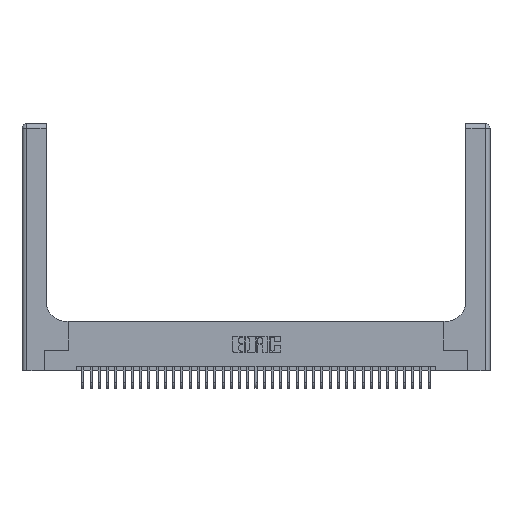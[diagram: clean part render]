
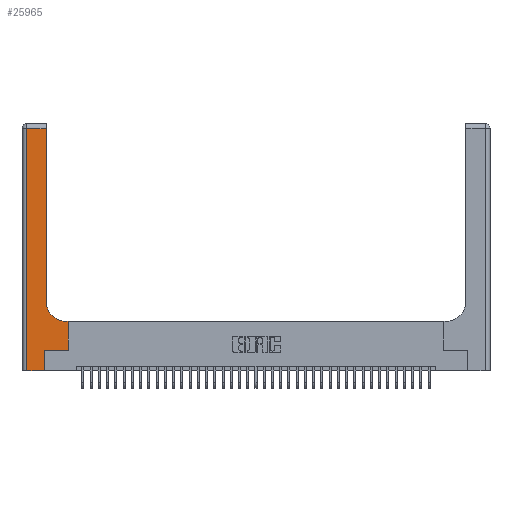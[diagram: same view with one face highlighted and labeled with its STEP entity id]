
A CAD part, top view. The second image highlights one B-rep face of the part: STEP entity #25965.
In plain terms, the highlighted planar face has unit normal (0, 0, 1).
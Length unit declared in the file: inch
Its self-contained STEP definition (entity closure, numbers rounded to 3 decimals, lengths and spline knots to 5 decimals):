
#508 = EDGE_CURVE ( 'NONE', #5268, #9219, #32286, .T. ) ;
#950 = EDGE_CURVE ( 'NONE', #16407, #36131, #2980, .T. ) ;
#1667 = EDGE_LOOP ( 'NONE', ( #16238, #14206, #35951, #24288, #27213, #13614, #34308, #2394, #36079 ) ) ;
#1693 = EDGE_CURVE ( 'NONE', #23005, #19528, #11734, .T. ) ;
#1925 = CARTESIAN_POINT ( 'NONE',  ( 0.269, 0., 0.37 ) ) ;
#2394 = ORIENTED_EDGE ( 'NONE', *, *, #508, .T. ) ;
#2980 = LINE ( 'NONE', #14842, #29808 ) ;
#3541 = CARTESIAN_POINT ( 'NONE',  ( 0.269, 0.25, 0.37 ) ) ;
#5268 = VERTEX_POINT ( 'NONE', #5481 ) ;
#5481 = CARTESIAN_POINT ( 'NONE',  ( 0.5585, 0.6, 0.37 ) ) ;
#6613 = LINE ( 'NONE', #32759, #22176 ) ;
#6813 = VECTOR ( 'NONE', #40190, 39.37008 ) ;
#7052 = CARTESIAN_POINT ( 'NONE',  ( 0.269, 0., 0.37 ) ) ;
#7204 = VECTOR ( 'NONE', #33166, 39.37008 ) ;
#7894 = CARTESIAN_POINT ( 'NONE',  ( 0.5585, 0.25, 0.37 ) ) ;
#8681 = LINE ( 'NONE', #14124, #11570 ) ;
#8994 = FACE_OUTER_BOUND ( 'NONE', #1667, .T. ) ;
#9185 = CARTESIAN_POINT ( 'NONE',  ( 0.2915, 0.85, 0.37 ) ) ;
#9219 = VERTEX_POINT ( 'NONE', #16003 ) ;
#9409 = DIRECTION ( 'NONE',  ( 1., 0., 0. ) ) ;
#9759 = EDGE_CURVE ( 'NONE', #36131, #5268, #8681, .T. ) ;
#10856 = DIRECTION ( 'NONE',  ( 0., 1., 0. ) ) ;
#11108 = CARTESIAN_POINT ( 'NONE',  ( 0.06, 0., 0.37 ) ) ;
#11570 = VECTOR ( 'NONE', #10856, 39.37008 ) ;
#11590 = CARTESIAN_POINT ( 'NONE',  ( 0.06, 2.94, 0.37 ) ) ;
#11734 = LINE ( 'NONE', #12444, #6813 ) ;
#12444 = CARTESIAN_POINT ( 'NONE',  ( 0., 0., 0.37 ) ) ;
#12936 = DIRECTION ( 'NONE',  ( -1., 0., 0. ) ) ;
#13614 = ORIENTED_EDGE ( 'NONE', *, *, #950, .T. ) ;
#13839 = AXIS2_PLACEMENT_3D ( 'NONE', #16991, #38860, #35831 ) ;
#14124 = CARTESIAN_POINT ( 'NONE',  ( 0.5585, 0.25, 0.37 ) ) ;
#14206 = ORIENTED_EDGE ( 'NONE', *, *, #31588, .T. ) ;
#14261 = CARTESIAN_POINT ( 'NONE',  ( 0.2915, 0.6, 0.37 ) ) ;
#14512 = LINE ( 'NONE', #1925, #7204 ) ;
#14842 = CARTESIAN_POINT ( 'NONE',  ( 0.269, 0.25, 0.37 ) ) ;
#15973 = VERTEX_POINT ( 'NONE', #11590 ) ;
#15982 = EDGE_CURVE ( 'NONE', #19528, #16407, #14512, .T. ) ;
#16003 = CARTESIAN_POINT ( 'NONE',  ( 0.5415, 0.6, 0.37 ) ) ;
#16238 = ORIENTED_EDGE ( 'NONE', *, *, #31665, .T. ) ;
#16407 = VERTEX_POINT ( 'NONE', #3541 ) ;
#16991 = CARTESIAN_POINT ( 'NONE',  ( 0.5415, 0.85, 0.37 ) ) ;
#17520 = VERTEX_POINT ( 'NONE', #24268 ) ;
#19086 = EDGE_CURVE ( 'NONE', #9219, #24053, #21640, .T. ) ;
#19528 = VERTEX_POINT ( 'NONE', #7052 ) ;
#21524 = DIRECTION ( 'NONE',  ( 0., 1., 0. ) ) ;
#21640 = CIRCLE ( 'NONE', #13839, 0.25 ) ;
#22080 = DIRECTION ( 'NONE',  ( 0., -1., 0. ) ) ;
#22176 = VECTOR ( 'NONE', #32898, 39.37008 ) ;
#23005 = VERTEX_POINT ( 'NONE', #11108 ) ;
#24053 = VERTEX_POINT ( 'NONE', #9185 ) ;
#24268 = CARTESIAN_POINT ( 'NONE',  ( 0.2915, 2.94, 0.37 ) ) ;
#24288 = ORIENTED_EDGE ( 'NONE', *, *, #1693, .T. ) ;
#25965 = ADVANCED_FACE ( 'NONE', ( #8994 ), #27673, .F. ) ;
#27213 = ORIENTED_EDGE ( 'NONE', *, *, #15982, .T. ) ;
#27673 = PLANE ( 'NONE',  #36838 ) ;
#29808 = VECTOR ( 'NONE', #9409, 39.37008 ) ;
#29972 = VECTOR ( 'NONE', #21524, 39.37008 ) ;
#31588 = EDGE_CURVE ( 'NONE', #17520, #15973, #6613, .T. ) ;
#31665 = EDGE_CURVE ( 'NONE', #24053, #17520, #33417, .T. ) ;
#31674 = CARTESIAN_POINT ( 'NONE',  ( 0.06, 3., 0.37 ) ) ;
#32043 = DIRECTION ( 'NONE',  ( 0., 0., -1. ) ) ;
#32286 = LINE ( 'NONE', #14261, #36231 ) ;
#32759 = CARTESIAN_POINT ( 'NONE',  ( 0., 2.94, 0.37 ) ) ;
#32898 = DIRECTION ( 'NONE',  ( -1., 0., 0. ) ) ;
#33166 = DIRECTION ( 'NONE',  ( 0., 1., 0. ) ) ;
#33417 = LINE ( 'NONE', #39185, #29972 ) ;
#34308 = ORIENTED_EDGE ( 'NONE', *, *, #9759, .T. ) ;
#35262 = EDGE_CURVE ( 'NONE', #15973, #23005, #36877, .T. ) ;
#35831 = DIRECTION ( 'NONE',  ( 1., 0., 0. ) ) ;
#35951 = ORIENTED_EDGE ( 'NONE', *, *, #35262, .T. ) ;
#36079 = ORIENTED_EDGE ( 'NONE', *, *, #19086, .T. ) ;
#36131 = VERTEX_POINT ( 'NONE', #7894 ) ;
#36231 = VECTOR ( 'NONE', #39278, 39.37008 ) ;
#36838 = AXIS2_PLACEMENT_3D ( 'NONE', #38067, #32043, #12936 ) ;
#36877 = LINE ( 'NONE', #31674, #37852 ) ;
#37852 = VECTOR ( 'NONE', #22080, 39.37008 ) ;
#38067 = CARTESIAN_POINT ( 'NONE',  ( 0., 3., 0.37 ) ) ;
#38860 = DIRECTION ( 'NONE',  ( 0., 0., -1. ) ) ;
#39185 = CARTESIAN_POINT ( 'NONE',  ( 0.2915, 3., 0.37 ) ) ;
#39278 = DIRECTION ( 'NONE',  ( -1., 0., 0. ) ) ;
#40190 = DIRECTION ( 'NONE',  ( 1., 0., 0. ) ) ;
